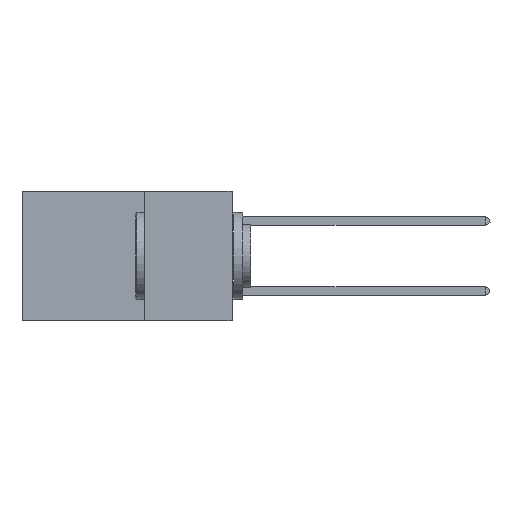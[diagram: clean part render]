
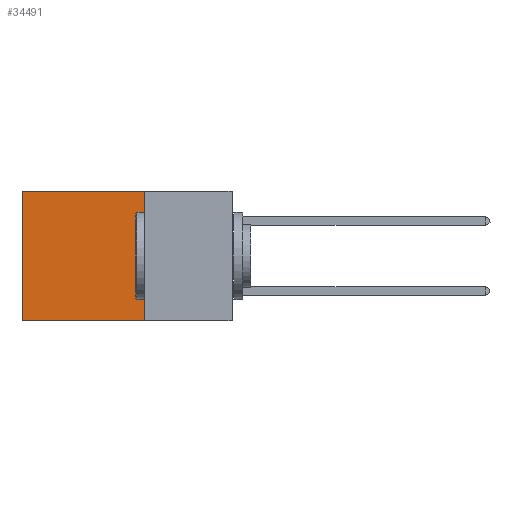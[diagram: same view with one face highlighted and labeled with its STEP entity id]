
A CAD part, left-side view. The second image highlights one B-rep face of the part: STEP entity #34491.
In plain terms, the highlighted planar face has unit normal (-1, 0, 0).
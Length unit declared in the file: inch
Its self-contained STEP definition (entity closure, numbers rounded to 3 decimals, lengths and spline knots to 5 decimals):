
#422 = CARTESIAN_POINT ( 'NONE',  ( 0.2875, 0.25, -0.37 ) ) ;
#576 = CARTESIAN_POINT ( 'NONE',  ( 0.2875, 0.6, -0.37 ) ) ;
#1977 = CARTESIAN_POINT ( 'NONE',  ( 0.2875, 0.25, 0. ) ) ;
#2963 = CARTESIAN_POINT ( 'NONE',  ( 0.2875, 0.25, 0. ) ) ;
#3682 = VECTOR ( 'NONE', #27385, 39.37008 ) ;
#4278 = CARTESIAN_POINT ( 'NONE',  ( 0.2875, 0.25, -0.37 ) ) ;
#8660 = CARTESIAN_POINT ( 'NONE',  ( 0.2875, 0.6, 0. ) ) ;
#9818 = VECTOR ( 'NONE', #20757, 39.37008 ) ;
#11207 = LINE ( 'NONE', #2963, #27751 ) ;
#12784 = LINE ( 'NONE', #8660, #37988 ) ;
#12891 = VERTEX_POINT ( 'NONE', #1977 ) ;
#13239 = DIRECTION ( 'NONE',  ( 1., 0., 0. ) ) ;
#15135 = VERTEX_POINT ( 'NONE', #576 ) ;
#17784 = EDGE_CURVE ( 'NONE', #12891, #36713, #11207, .T. ) ;
#20757 = DIRECTION ( 'NONE',  ( 0., 1., 0. ) ) ;
#21803 = EDGE_LOOP ( 'NONE', ( #36356, #28809, #29839, #28407 ) ) ;
#22456 = CARTESIAN_POINT ( 'NONE',  ( 0.2875, 0.6, 0. ) ) ;
#23731 = EDGE_CURVE ( 'NONE', #12891, #34361, #26396, .T. ) ;
#24476 = FACE_OUTER_BOUND ( 'NONE', #21803, .T. ) ;
#26340 = PLANE ( 'NONE',  #38839 ) ;
#26396 = LINE ( 'NONE', #40373, #9818 ) ;
#27385 = DIRECTION ( 'NONE',  ( 0., 1., 0. ) ) ;
#27751 = VECTOR ( 'NONE', #42350, 39.37008 ) ;
#28407 = ORIENTED_EDGE ( 'NONE', *, *, #23731, .T. ) ;
#28809 = ORIENTED_EDGE ( 'NONE', *, *, #35504, .F. ) ;
#29839 = ORIENTED_EDGE ( 'NONE', *, *, #17784, .F. ) ;
#32944 = CARTESIAN_POINT ( 'NONE',  ( 0.2875, 0.25, 0. ) ) ;
#34361 = VERTEX_POINT ( 'NONE', #22456 ) ;
#34491 = ADVANCED_FACE ( 'NONE', ( #24476 ), #26340, .F. ) ;
#35067 = DIRECTION ( 'NONE',  ( 0., 0., -1. ) ) ;
#35504 = EDGE_CURVE ( 'NONE', #36713, #15135, #38747, .T. ) ;
#36226 = DIRECTION ( 'NONE',  ( 0., 0., -1. ) ) ;
#36356 = ORIENTED_EDGE ( 'NONE', *, *, #42358, .T. ) ;
#36713 = VERTEX_POINT ( 'NONE', #422 ) ;
#37988 = VECTOR ( 'NONE', #35067, 39.37008 ) ;
#38747 = LINE ( 'NONE', #4278, #3682 ) ;
#38839 = AXIS2_PLACEMENT_3D ( 'NONE', #32944, #13239, #36226 ) ;
#40373 = CARTESIAN_POINT ( 'NONE',  ( 0.2875, 0.25, 0. ) ) ;
#42350 = DIRECTION ( 'NONE',  ( 0., 0., -1. ) ) ;
#42358 = EDGE_CURVE ( 'NONE', #34361, #15135, #12784, .T. ) ;
